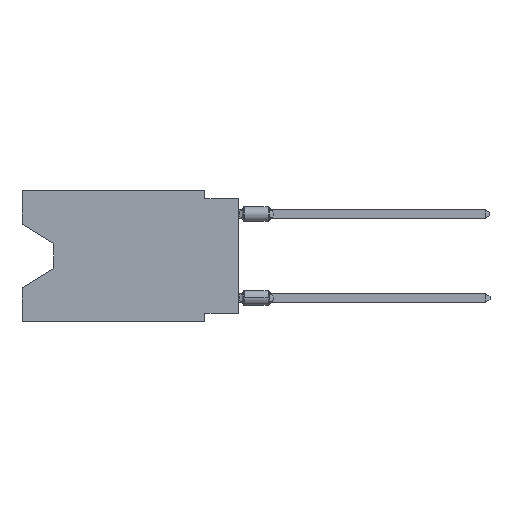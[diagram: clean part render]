
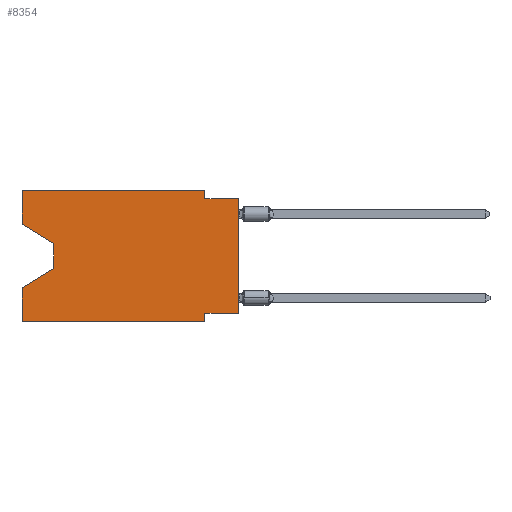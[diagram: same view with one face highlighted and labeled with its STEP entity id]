
A CAD part, left-side view. The second image highlights one B-rep face of the part: STEP entity #8354.
In plain terms, the highlighted planar face has unit normal (-1, 0, 0).
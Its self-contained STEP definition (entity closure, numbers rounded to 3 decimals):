
#128 = VECTOR ( 'NONE', #3364, 1000. ) ;
#548 = LINE ( 'NONE', #9732, #28758 ) ;
#639 = EDGE_CURVE ( 'NONE', #13445, #15237, #23978, .T. ) ;
#700 = ORIENTED_EDGE ( 'NONE', *, *, #1523, .F. ) ;
#794 = AXIS2_PLACEMENT_3D ( 'NONE', #3652, #17031, #19460 ) ;
#1152 = VERTEX_POINT ( 'NONE', #12881 ) ;
#1162 = CARTESIAN_POINT ( 'NONE',  ( 0., 0., -0.635 ) ) ;
#1523 = EDGE_CURVE ( 'NONE', #21747, #13553, #26029, .T. ) ;
#1810 = EDGE_LOOP ( 'NONE', ( #29561, #23151, #28609, #6069, #14405, #21680, #10954, #18953, #700, #19512, #20042, #25974 ) ) ;
#2081 = CARTESIAN_POINT ( 'NONE',  ( 0., 16.383, 0. ) ) ;
#2656 = DIRECTION ( 'NONE',  ( 0., 0., -1. ) ) ;
#3134 = EDGE_CURVE ( 'NONE', #21718, #21747, #28868, .T. ) ;
#3157 = CARTESIAN_POINT ( 'NONE',  ( 0., 0., -0.635 ) ) ;
#3364 = DIRECTION ( 'NONE',  ( 0., 0.855, -0.519 ) ) ;
#3584 = DIRECTION ( 'NONE',  ( 0., 1., 0. ) ) ;
#3652 = CARTESIAN_POINT ( 'NONE',  ( 0., 16.383, 0. ) ) ;
#4636 = LINE ( 'NONE', #6577, #19012 ) ;
#5111 = VERTEX_POINT ( 'NONE', #28088 ) ;
#6043 = EDGE_CURVE ( 'NONE', #29409, #13553, #18184, .T. ) ;
#6069 = ORIENTED_EDGE ( 'NONE', *, *, #639, .F. ) ;
#6577 = CARTESIAN_POINT ( 'NONE',  ( 0., 2.54, -9.906 ) ) ;
#6614 = CARTESIAN_POINT ( 'NONE',  ( 0., 0., -9.271 ) ) ;
#7320 = EDGE_CURVE ( 'NONE', #14107, #23906, #4636, .T. ) ;
#7908 = LINE ( 'NONE', #21952, #24803 ) ;
#8049 = VECTOR ( 'NONE', #11549, 1000. ) ;
#8201 = DIRECTION ( 'NONE',  ( 0., 0., -1. ) ) ;
#8354 = ADVANCED_FACE ( 'NONE', ( #28217 ), #26101, .F. ) ;
#9010 = DIRECTION ( 'NONE',  ( 0., 0., -1. ) ) ;
#9732 = CARTESIAN_POINT ( 'NONE',  ( 0., 13.97, -4.013 ) ) ;
#10026 = VECTOR ( 'NONE', #8201, 1000. ) ;
#10334 = CARTESIAN_POINT ( 'NONE',  ( 0., 2.54, -9.271 ) ) ;
#10535 = CARTESIAN_POINT ( 'NONE',  ( 0., 2.54, -9.906 ) ) ;
#10954 = ORIENTED_EDGE ( 'NONE', *, *, #26686, .F. ) ;
#10963 = CARTESIAN_POINT ( 'NONE',  ( 0., 0., 0. ) ) ;
#11549 = DIRECTION ( 'NONE',  ( 0., 0., 1. ) ) ;
#11591 = CARTESIAN_POINT ( 'NONE',  ( 0., 16.383, -9.906 ) ) ;
#12383 = LINE ( 'NONE', #14078, #26967 ) ;
#12390 = CARTESIAN_POINT ( 'NONE',  ( 0., 2.54, -0.635 ) ) ;
#12855 = VECTOR ( 'NONE', #21278, 1000. ) ;
#12881 = CARTESIAN_POINT ( 'NONE',  ( 0., 13.97, -4.013 ) ) ;
#13023 = CARTESIAN_POINT ( 'NONE',  ( 0., 2.54, 0. ) ) ;
#13412 = LINE ( 'NONE', #22626, #18250 ) ;
#13445 = VERTEX_POINT ( 'NONE', #11591 ) ;
#13553 = VERTEX_POINT ( 'NONE', #3157 ) ;
#14078 = CARTESIAN_POINT ( 'NONE',  ( 0., 16.383, -9.906 ) ) ;
#14107 = VERTEX_POINT ( 'NONE', #10334 ) ;
#14405 = ORIENTED_EDGE ( 'NONE', *, *, #20406, .T. ) ;
#14650 = CARTESIAN_POINT ( 'NONE',  ( 0., 13.97, -5.893 ) ) ;
#14888 = LINE ( 'NONE', #29056, #26979 ) ;
#15008 = DIRECTION ( 'NONE',  ( 0., -1., 0. ) ) ;
#15237 = VERTEX_POINT ( 'NONE', #27753 ) ;
#15791 = LINE ( 'NONE', #2081, #8049 ) ;
#16203 = EDGE_CURVE ( 'NONE', #5111, #15237, #28667, .T. ) ;
#16475 = DIRECTION ( 'NONE',  ( 0., -1., 0. ) ) ;
#16773 = CARTESIAN_POINT ( 'NONE',  ( 0., 16.383, -2.546 ) ) ;
#17031 = DIRECTION ( 'NONE',  ( 1., 0., 0. ) ) ;
#17902 = CARTESIAN_POINT ( 'NONE',  ( 0., 16.383, 0. ) ) ;
#18160 = EDGE_CURVE ( 'NONE', #1152, #5111, #548, .T. ) ;
#18184 = LINE ( 'NONE', #10963, #19942 ) ;
#18250 = VECTOR ( 'NONE', #29563, 1000. ) ;
#18336 = DIRECTION ( 'NONE',  ( 0., 0., 1. ) ) ;
#18953 = ORIENTED_EDGE ( 'NONE', *, *, #6043, .T. ) ;
#19012 = VECTOR ( 'NONE', #9010, 1000. ) ;
#19460 = DIRECTION ( 'NONE',  ( 0., 0., -1. ) ) ;
#19512 = ORIENTED_EDGE ( 'NONE', *, *, #3134, .F. ) ;
#19534 = DIRECTION ( 'NONE',  ( 0., -1., 0. ) ) ;
#19535 = EDGE_CURVE ( 'NONE', #24111, #21718, #7908, .T. ) ;
#19942 = VECTOR ( 'NONE', #18336, 1000. ) ;
#20042 = ORIENTED_EDGE ( 'NONE', *, *, #19535, .F. ) ;
#20406 = EDGE_CURVE ( 'NONE', #13445, #23906, #12383, .T. ) ;
#21115 = EDGE_CURVE ( 'NONE', #28772, #24111, #15791, .T. ) ;
#21126 = VECTOR ( 'NONE', #19534, 1000. ) ;
#21278 = DIRECTION ( 'NONE',  ( 0., 0., 1. ) ) ;
#21680 = ORIENTED_EDGE ( 'NONE', *, *, #7320, .F. ) ;
#21718 = VERTEX_POINT ( 'NONE', #25987 ) ;
#21747 = VERTEX_POINT ( 'NONE', #12390 ) ;
#21952 = CARTESIAN_POINT ( 'NONE',  ( 0., 16.383, 0. ) ) ;
#22626 = CARTESIAN_POINT ( 'NONE',  ( 0., 16.383, -2.546 ) ) ;
#23151 = ORIENTED_EDGE ( 'NONE', *, *, #18160, .T. ) ;
#23906 = VERTEX_POINT ( 'NONE', #10535 ) ;
#23978 = LINE ( 'NONE', #26086, #12855 ) ;
#24111 = VERTEX_POINT ( 'NONE', #17902 ) ;
#24803 = VECTOR ( 'NONE', #15008, 1000. ) ;
#25974 = ORIENTED_EDGE ( 'NONE', *, *, #21115, .F. ) ;
#25987 = CARTESIAN_POINT ( 'NONE',  ( 0., 2.54, 0. ) ) ;
#26029 = LINE ( 'NONE', #1162, #21126 ) ;
#26086 = CARTESIAN_POINT ( 'NONE',  ( 0., 16.383, 0. ) ) ;
#26101 = PLANE ( 'NONE',  #794 ) ;
#26686 = EDGE_CURVE ( 'NONE', #29409, #14107, #14888, .T. ) ;
#26967 = VECTOR ( 'NONE', #16475, 1000. ) ;
#26979 = VECTOR ( 'NONE', #3584, 1000. ) ;
#27753 = CARTESIAN_POINT ( 'NONE',  ( 0., 16.383, -7.36 ) ) ;
#28088 = CARTESIAN_POINT ( 'NONE',  ( 0., 13.97, -5.893 ) ) ;
#28217 = FACE_OUTER_BOUND ( 'NONE', #1810, .T. ) ;
#28609 = ORIENTED_EDGE ( 'NONE', *, *, #16203, .T. ) ;
#28667 = LINE ( 'NONE', #14650, #128 ) ;
#28758 = VECTOR ( 'NONE', #2656, 1000. ) ;
#28772 = VERTEX_POINT ( 'NONE', #16773 ) ;
#28868 = LINE ( 'NONE', #13023, #10026 ) ;
#29056 = CARTESIAN_POINT ( 'NONE',  ( 0., 0., -9.271 ) ) ;
#29409 = VERTEX_POINT ( 'NONE', #6614 ) ;
#29503 = EDGE_CURVE ( 'NONE', #28772, #1152, #13412, .T. ) ;
#29561 = ORIENTED_EDGE ( 'NONE', *, *, #29503, .T. ) ;
#29563 = DIRECTION ( 'NONE',  ( 0., -0.855, -0.519 ) ) ;
